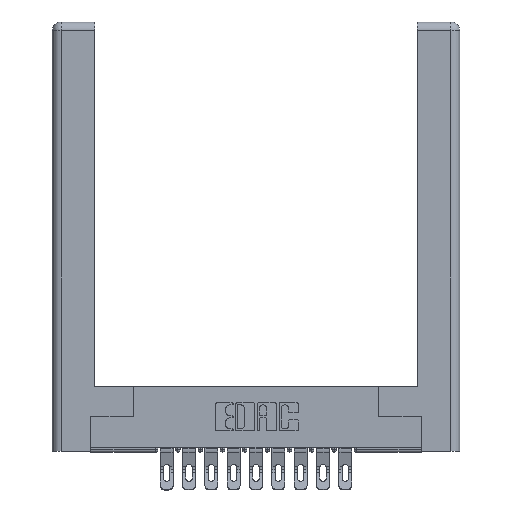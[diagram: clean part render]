
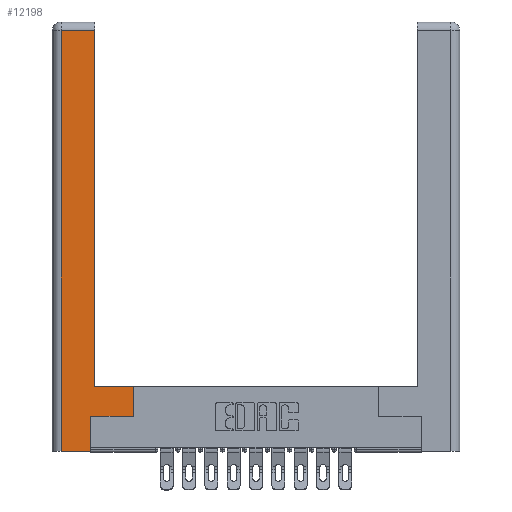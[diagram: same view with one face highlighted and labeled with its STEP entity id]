
A CAD part, top view. The second image highlights one B-rep face of the part: STEP entity #12198.
In plain terms, the highlighted planar face has unit normal (0, 0, 1).
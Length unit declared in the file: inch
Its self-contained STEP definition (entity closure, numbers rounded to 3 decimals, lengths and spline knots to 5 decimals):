
#152 = DIRECTION ( 'NONE',  ( -1., 0., 0. ) ) ;
#218 = VERTEX_POINT ( 'NONE', #4839 ) ;
#220 = LINE ( 'NONE', #14343, #14225 ) ;
#302 = LINE ( 'NONE', #6370, #13882 ) ;
#336 = VERTEX_POINT ( 'NONE', #5122 ) ;
#457 = ORIENTED_EDGE ( 'NONE', *, *, #12117, .T. ) ;
#956 = DIRECTION ( 'NONE',  ( 1., 0., 0. ) ) ;
#1244 = VERTEX_POINT ( 'NONE', #9947 ) ;
#2214 = CARTESIAN_POINT ( 'NONE',  ( 0.565, 0.245, 0. ) ) ;
#2232 = CARTESIAN_POINT ( 'NONE',  ( 0.265, 0.245, 0. ) ) ;
#2249 = VECTOR ( 'NONE', #956, 39.37008 ) ;
#2598 = ORIENTED_EDGE ( 'NONE', *, *, #7455, .T. ) ;
#2663 = VECTOR ( 'NONE', #152, 39.37008 ) ;
#2666 = EDGE_CURVE ( 'NONE', #3279, #11262, #12312, .T. ) ;
#3279 = VERTEX_POINT ( 'NONE', #6739 ) ;
#3625 = CARTESIAN_POINT ( 'NONE',  ( 0.295, 0.45, 0. ) ) ;
#3847 = VECTOR ( 'NONE', #14109, 39.37008 ) ;
#4020 = CARTESIAN_POINT ( 'NONE',  ( 0.0615, 2.94, 0. ) ) ;
#4040 = LINE ( 'NONE', #2232, #3847 ) ;
#4136 = ORIENTED_EDGE ( 'NONE', *, *, #6167, .T. ) ;
#4353 = DIRECTION ( 'NONE',  ( 0., -1., 0. ) ) ;
#4670 = CARTESIAN_POINT ( 'NONE',  ( 0.0615, 2.94, 0. ) ) ;
#4839 = CARTESIAN_POINT ( 'NONE',  ( 0.565, 0.45, 0. ) ) ;
#4987 = ORIENTED_EDGE ( 'NONE', *, *, #9711, .T. ) ;
#5006 = EDGE_LOOP ( 'NONE', ( #15270, #5383, #2598, #16646, #11729, #4136, #4987, #457 ) ) ;
#5122 = CARTESIAN_POINT ( 'NONE',  ( 0.265, 0.245, 0. ) ) ;
#5182 = LINE ( 'NONE', #16604, #8760 ) ;
#5383 = ORIENTED_EDGE ( 'NONE', *, *, #2666, .T. ) ;
#5439 = CARTESIAN_POINT ( 'NONE',  ( 0., 0., 0. ) ) ;
#5715 = LINE ( 'NONE', #2214, #2249 ) ;
#6167 = EDGE_CURVE ( 'NONE', #336, #13103, #5715, .T. ) ;
#6370 = CARTESIAN_POINT ( 'NONE',  ( 0.265, 0., 0. ) ) ;
#6739 = CARTESIAN_POINT ( 'NONE',  ( 0.295, 2.94, 0. ) ) ;
#6830 = DIRECTION ( 'NONE',  ( -1., 0., 0. ) ) ;
#7185 = AXIS2_PLACEMENT_3D ( 'NONE', #5439, #8189, #6830 ) ;
#7455 = EDGE_CURVE ( 'NONE', #11262, #1244, #16652, .T. ) ;
#7518 = FACE_OUTER_BOUND ( 'NONE', #5006, .T. ) ;
#7536 = VECTOR ( 'NONE', #16946, 39.37008 ) ;
#7753 = DIRECTION ( 'NONE',  ( 0., 1., 0. ) ) ;
#7847 = CARTESIAN_POINT ( 'NONE',  ( 0.0615, 0., 0. ) ) ;
#8189 = DIRECTION ( 'NONE',  ( 0., 0., -1. ) ) ;
#8228 = CARTESIAN_POINT ( 'NONE',  ( 0.265, 0., 0. ) ) ;
#8380 = LINE ( 'NONE', #13021, #7536 ) ;
#8760 = VECTOR ( 'NONE', #9858, 39.37008 ) ;
#9711 = EDGE_CURVE ( 'NONE', #13103, #218, #5182, .T. ) ;
#9858 = DIRECTION ( 'NONE',  ( 0., 1., 0. ) ) ;
#9947 = CARTESIAN_POINT ( 'NONE',  ( 0.0615, 0., 0. ) ) ;
#9992 = VERTEX_POINT ( 'NONE', #3625 ) ;
#10486 = DIRECTION ( 'NONE',  ( 1., 0., 0. ) ) ;
#11262 = VERTEX_POINT ( 'NONE', #4670 ) ;
#11293 = EDGE_CURVE ( 'NONE', #13637, #336, #4040, .T. ) ;
#11729 = ORIENTED_EDGE ( 'NONE', *, *, #11293, .T. ) ;
#12117 = EDGE_CURVE ( 'NONE', #218, #9992, #8380, .T. ) ;
#12198 = ADVANCED_FACE ( 'NONE', ( #7518 ), #14711, .F. ) ;
#12312 = LINE ( 'NONE', #4020, #2663 ) ;
#13021 = CARTESIAN_POINT ( 'NONE',  ( 0.295, 0.45, 0. ) ) ;
#13103 = VERTEX_POINT ( 'NONE', #16952 ) ;
#13456 = EDGE_CURVE ( 'NONE', #1244, #13637, #302, .T. ) ;
#13637 = VERTEX_POINT ( 'NONE', #8228 ) ;
#13882 = VECTOR ( 'NONE', #10486, 39.37008 ) ;
#14109 = DIRECTION ( 'NONE',  ( 0., 1., 0. ) ) ;
#14225 = VECTOR ( 'NONE', #7753, 39.37008 ) ;
#14343 = CARTESIAN_POINT ( 'NONE',  ( 0.295, 3., 0. ) ) ;
#14711 = PLANE ( 'NONE',  #7185 ) ;
#15270 = ORIENTED_EDGE ( 'NONE', *, *, #16334, .T. ) ;
#15827 = VECTOR ( 'NONE', #4353, 39.37008 ) ;
#16334 = EDGE_CURVE ( 'NONE', #9992, #3279, #220, .T. ) ;
#16604 = CARTESIAN_POINT ( 'NONE',  ( 0.565, 0.45, 0. ) ) ;
#16646 = ORIENTED_EDGE ( 'NONE', *, *, #13456, .T. ) ;
#16652 = LINE ( 'NONE', #7847, #15827 ) ;
#16946 = DIRECTION ( 'NONE',  ( -1., 0., 0. ) ) ;
#16952 = CARTESIAN_POINT ( 'NONE',  ( 0.565, 0.245, 0. ) ) ;
